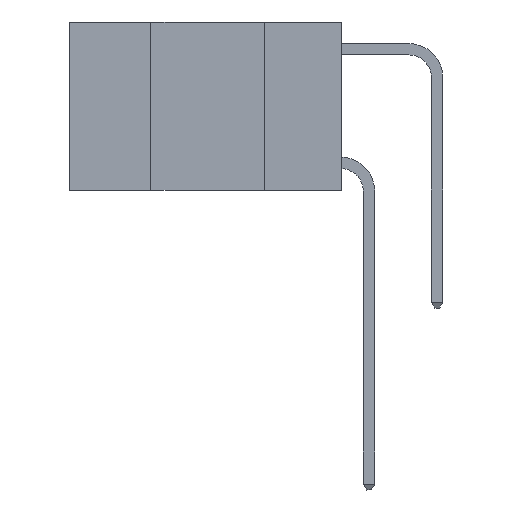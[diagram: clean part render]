
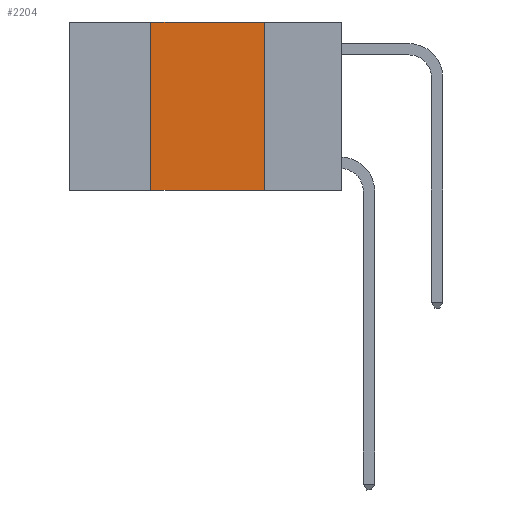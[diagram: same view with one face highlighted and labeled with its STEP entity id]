
A CAD part, left-side view. The second image highlights one B-rep face of the part: STEP entity #2204.
In plain terms, the highlighted planar face has unit normal (-1, 0, 0).
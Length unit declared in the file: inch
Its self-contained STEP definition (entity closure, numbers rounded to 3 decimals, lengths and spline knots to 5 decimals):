
#55 = ORIENTED_EDGE ( 'NONE', *, *, #6683, .F. ) ;
#305 = AXIS2_PLACEMENT_3D ( 'NONE', #7136, #10332, #7858 ) ;
#661 = CARTESIAN_POINT ( 'NONE',  ( 0., 0.17, 0. ) ) ;
#945 = EDGE_LOOP ( 'NONE', ( #55, #1006, #2959, #7457 ) ) ;
#1006 = ORIENTED_EDGE ( 'NONE', *, *, #4513, .F. ) ;
#1240 = LINE ( 'NONE', #9963, #5965 ) ;
#2028 = LINE ( 'NONE', #2815, #11129 ) ;
#2204 = ADVANCED_FACE ( 'NONE', ( #3058 ), #8363, .F. ) ;
#2459 = CARTESIAN_POINT ( 'NONE',  ( 0., 0.42, 0. ) ) ;
#2815 = CARTESIAN_POINT ( 'NONE',  ( 0., 0.6, -0.37 ) ) ;
#2959 = ORIENTED_EDGE ( 'NONE', *, *, #7819, .F. ) ;
#3058 = FACE_OUTER_BOUND ( 'NONE', #945, .T. ) ;
#3330 = VECTOR ( 'NONE', #4123, 39.37008 ) ;
#3844 = VERTEX_POINT ( 'NONE', #11090 ) ;
#4123 = DIRECTION ( 'NONE',  ( 0., -1., 0. ) ) ;
#4502 = LINE ( 'NONE', #9657, #11043 ) ;
#4513 = EDGE_CURVE ( 'NONE', #8877, #6786, #8216, .T. ) ;
#5888 = VERTEX_POINT ( 'NONE', #11346 ) ;
#5965 = VECTOR ( 'NONE', #10796, 39.37008 ) ;
#6404 = DIRECTION ( 'NONE',  ( 0., -1., 0. ) ) ;
#6683 = EDGE_CURVE ( 'NONE', #6786, #5888, #4502, .T. ) ;
#6786 = VERTEX_POINT ( 'NONE', #661 ) ;
#7136 = CARTESIAN_POINT ( 'NONE',  ( 0., 0.6, 0. ) ) ;
#7457 = ORIENTED_EDGE ( 'NONE', *, *, #9118, .T. ) ;
#7819 = EDGE_CURVE ( 'NONE', #3844, #8877, #1240, .T. ) ;
#7858 = DIRECTION ( 'NONE',  ( 0., 0., -1. ) ) ;
#8216 = LINE ( 'NONE', #9286, #3330 ) ;
#8363 = PLANE ( 'NONE',  #305 ) ;
#8877 = VERTEX_POINT ( 'NONE', #2459 ) ;
#9118 = EDGE_CURVE ( 'NONE', #3844, #5888, #2028, .T. ) ;
#9286 = CARTESIAN_POINT ( 'NONE',  ( 0., 0.6, 0. ) ) ;
#9657 = CARTESIAN_POINT ( 'NONE',  ( 0., 0.17, 0. ) ) ;
#9963 = CARTESIAN_POINT ( 'NONE',  ( 0., 0.42, 0. ) ) ;
#10332 = DIRECTION ( 'NONE',  ( 1., 0., 0. ) ) ;
#10486 = DIRECTION ( 'NONE',  ( 0., 0., -1. ) ) ;
#10796 = DIRECTION ( 'NONE',  ( 0., 0., 1. ) ) ;
#11043 = VECTOR ( 'NONE', #10486, 39.37008 ) ;
#11090 = CARTESIAN_POINT ( 'NONE',  ( 0., 0.42, -0.37 ) ) ;
#11129 = VECTOR ( 'NONE', #6404, 39.37008 ) ;
#11346 = CARTESIAN_POINT ( 'NONE',  ( 0., 0.17, -0.37 ) ) ;
